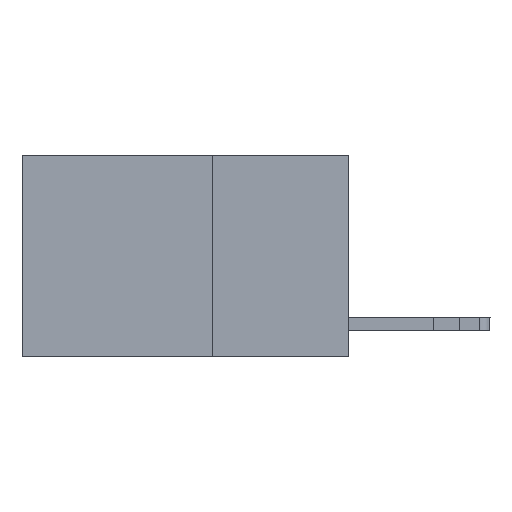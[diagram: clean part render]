
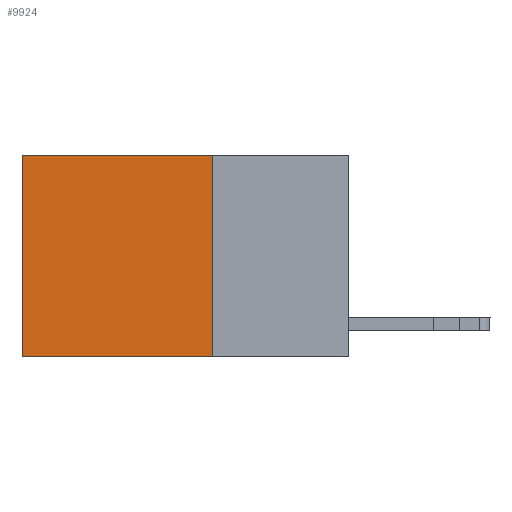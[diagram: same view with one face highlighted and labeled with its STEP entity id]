
A CAD part, left-side view. The second image highlights one B-rep face of the part: STEP entity #9924.
In plain terms, the highlighted planar face has unit normal (-1, 0, 0).
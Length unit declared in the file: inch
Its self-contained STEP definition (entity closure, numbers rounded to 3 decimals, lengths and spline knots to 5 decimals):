
#46 = CARTESIAN_POINT ( 'NONE',  ( 0.2625, 0.6, 0. ) ) ;
#244 = EDGE_CURVE ( 'NONE', #16210, #18952, #17261, .T. ) ;
#1495 = ORIENTED_EDGE ( 'NONE', *, *, #244, .T. ) ;
#3126 = VERTEX_POINT ( 'NONE', #15880 ) ;
#3142 = CARTESIAN_POINT ( 'NONE',  ( 0.2625, 0.25, 0. ) ) ;
#3753 = LINE ( 'NONE', #17154, #15695 ) ;
#3844 = DIRECTION ( 'NONE',  ( 0., 0., -1. ) ) ;
#3956 = CARTESIAN_POINT ( 'NONE',  ( 0.2625, 0.25, 0. ) ) ;
#4967 = DIRECTION ( 'NONE',  ( 0., 0., -1. ) ) ;
#5084 = ORIENTED_EDGE ( 'NONE', *, *, #17467, .F. ) ;
#5504 = LINE ( 'NONE', #17746, #10514 ) ;
#6014 = AXIS2_PLACEMENT_3D ( 'NONE', #6619, #13787, #13887 ) ;
#6525 = PLANE ( 'NONE',  #6014 ) ;
#6619 = CARTESIAN_POINT ( 'NONE',  ( 0.2625, 0.25, 0. ) ) ;
#7840 = EDGE_CURVE ( 'NONE', #18952, #3126, #3753, .T. ) ;
#8632 = VERTEX_POINT ( 'NONE', #14054 ) ;
#9718 = EDGE_LOOP ( 'NONE', ( #11444, #5084, #19178, #1495 ) ) ;
#9747 = VECTOR ( 'NONE', #9858, 39.37008 ) ;
#9858 = DIRECTION ( 'NONE',  ( 0., 1., 0. ) ) ;
#9924 = ADVANCED_FACE ( 'NONE', ( #11170 ), #6525, .F. ) ;
#10514 = VECTOR ( 'NONE', #12982, 39.37008 ) ;
#11170 = FACE_OUTER_BOUND ( 'NONE', #9718, .T. ) ;
#11444 = ORIENTED_EDGE ( 'NONE', *, *, #7840, .T. ) ;
#11949 = LINE ( 'NONE', #13512, #14802 ) ;
#12982 = DIRECTION ( 'NONE',  ( 0., 1., 0. ) ) ;
#13512 = CARTESIAN_POINT ( 'NONE',  ( 0.2625, 0.25, 0. ) ) ;
#13787 = DIRECTION ( 'NONE',  ( 1., 0., 0. ) ) ;
#13887 = DIRECTION ( 'NONE',  ( 0., 0., -1. ) ) ;
#14054 = CARTESIAN_POINT ( 'NONE',  ( 0.2625, 0.25, -0.37 ) ) ;
#14802 = VECTOR ( 'NONE', #4967, 39.37008 ) ;
#14954 = EDGE_CURVE ( 'NONE', #16210, #8632, #11949, .T. ) ;
#15695 = VECTOR ( 'NONE', #3844, 39.37008 ) ;
#15880 = CARTESIAN_POINT ( 'NONE',  ( 0.2625, 0.6, -0.37 ) ) ;
#16210 = VERTEX_POINT ( 'NONE', #3142 ) ;
#17154 = CARTESIAN_POINT ( 'NONE',  ( 0.2625, 0.6, 0. ) ) ;
#17261 = LINE ( 'NONE', #3956, #9747 ) ;
#17467 = EDGE_CURVE ( 'NONE', #8632, #3126, #5504, .T. ) ;
#17746 = CARTESIAN_POINT ( 'NONE',  ( 0.2625, 0.25, -0.37 ) ) ;
#18952 = VERTEX_POINT ( 'NONE', #46 ) ;
#19178 = ORIENTED_EDGE ( 'NONE', *, *, #14954, .F. ) ;
